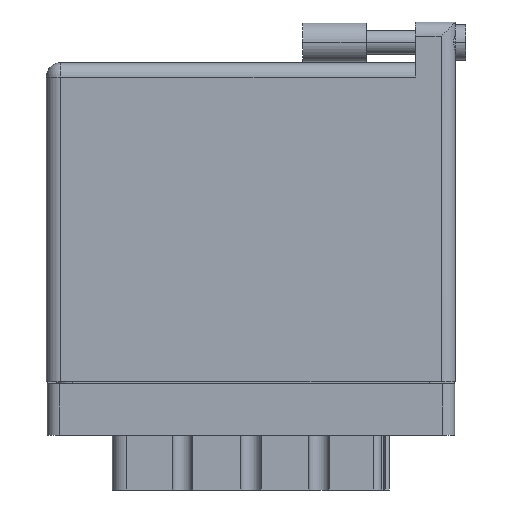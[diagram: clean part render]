
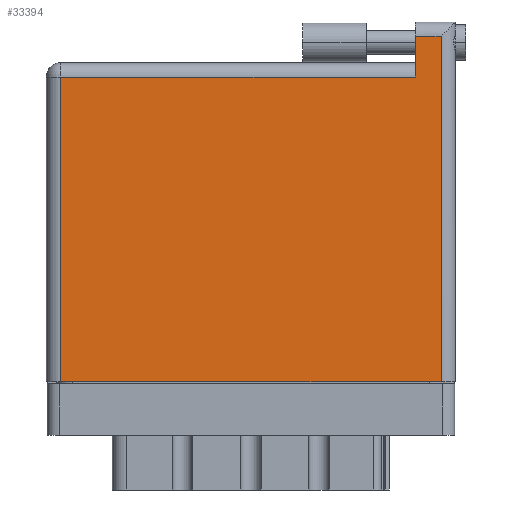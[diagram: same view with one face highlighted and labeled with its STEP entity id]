
A CAD part, front view. The second image highlights one B-rep face of the part: STEP entity #33394.
In plain terms, the highlighted face is planar.
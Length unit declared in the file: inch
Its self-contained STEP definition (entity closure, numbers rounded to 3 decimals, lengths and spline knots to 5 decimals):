
#1506 = DIRECTION ( 'NONE',  ( -1., 0., 0. ) ) ;
#2133 = CARTESIAN_POINT ( 'NONE',  ( 0.07, 0., 0. ) ) ;
#2409 = CARTESIAN_POINT ( 'NONE',  ( 0.07, 1.496, 0. ) ) ;
#3100 = AXIS2_PLACEMENT_3D ( 'NONE', #13180, #16184, #10576 ) ;
#3564 = VERTEX_POINT ( 'NONE', #29487 ) ;
#3925 = VECTOR ( 'NONE', #17186, 39.37008 ) ;
#4521 = ORIENTED_EDGE ( 'NONE', *, *, #5696, .T. ) ;
#5093 = CARTESIAN_POINT ( 'NONE',  ( 1.811, 1.766, 0. ) ) ;
#5696 = EDGE_CURVE ( 'NONE', #34384, #31075, #9668, .T. ) ;
#5845 = VERTEX_POINT ( 'NONE', #22641 ) ;
#6347 = VECTOR ( 'NONE', #23750, 39.37008 ) ;
#7168 = DIRECTION ( 'NONE',  ( -1., 0., 0. ) ) ;
#7696 = VECTOR ( 'NONE', #31211, 39.37008 ) ;
#9415 = VECTOR ( 'NONE', #7168, 39.37008 ) ;
#9668 = LINE ( 'NONE', #19172, #15925 ) ;
#10206 = PLANE ( 'NONE',  #3100 ) ;
#10576 = DIRECTION ( 'NONE',  ( -1., 0., 0. ) ) ;
#13180 = CARTESIAN_POINT ( 'NONE',  ( 0., 1.566, 0. ) ) ;
#14721 = CARTESIAN_POINT ( 'NONE',  ( 1.938, 1.696, 0. ) ) ;
#14875 = LINE ( 'NONE', #24082, #33535 ) ;
#15925 = VECTOR ( 'NONE', #36089, 39.37008 ) ;
#16184 = DIRECTION ( 'NONE',  ( 0., 0., -1. ) ) ;
#17186 = DIRECTION ( 'NONE',  ( 1., 0., 0. ) ) ;
#19172 = CARTESIAN_POINT ( 'NONE',  ( 0.07, 0., 0. ) ) ;
#19460 = ORIENTED_EDGE ( 'NONE', *, *, #34209, .T. ) ;
#20539 = EDGE_CURVE ( 'NONE', #21911, #34384, #14875, .T. ) ;
#21175 = FACE_OUTER_BOUND ( 'NONE', #33820, .T. ) ;
#21911 = VERTEX_POINT ( 'NONE', #26838 ) ;
#22305 = VERTEX_POINT ( 'NONE', #14721 ) ;
#22641 = CARTESIAN_POINT ( 'NONE',  ( 1.938, 0., 0. ) ) ;
#22889 = LINE ( 'NONE', #5093, #7696 ) ;
#23346 = ORIENTED_EDGE ( 'NONE', *, *, #26032, .T. ) ;
#23750 = DIRECTION ( 'NONE',  ( 0., 1., 0. ) ) ;
#24021 = ORIENTED_EDGE ( 'NONE', *, *, #20539, .T. ) ;
#24082 = CARTESIAN_POINT ( 'NONE',  ( 0., 1.496, 0. ) ) ;
#25895 = CARTESIAN_POINT ( 'NONE',  ( 0., 0., 0. ) ) ;
#26032 = EDGE_CURVE ( 'NONE', #31075, #5845, #26668, .T. ) ;
#26668 = LINE ( 'NONE', #25895, #3925 ) ;
#26838 = CARTESIAN_POINT ( 'NONE',  ( 1.811, 1.496, 0. ) ) ;
#26971 = CARTESIAN_POINT ( 'NONE',  ( 1.938, 1.766, 0. ) ) ;
#28850 = ORIENTED_EDGE ( 'NONE', *, *, #34998, .T. ) ;
#29487 = CARTESIAN_POINT ( 'NONE',  ( 1.811, 1.696, 0. ) ) ;
#29806 = CARTESIAN_POINT ( 'NONE',  ( 0., 1.696, 0. ) ) ;
#30067 = LINE ( 'NONE', #26971, #6347 ) ;
#31075 = VERTEX_POINT ( 'NONE', #2133 ) ;
#31211 = DIRECTION ( 'NONE',  ( 0., -1., 0. ) ) ;
#33157 = ORIENTED_EDGE ( 'NONE', *, *, #35463, .T. ) ;
#33394 = ADVANCED_FACE ( 'NONE', ( #21175 ), #10206, .F. ) ;
#33535 = VECTOR ( 'NONE', #1506, 39.37008 ) ;
#33820 = EDGE_LOOP ( 'NONE', ( #23346, #19460, #33157, #28850, #24021, #4521 ) ) ;
#34209 = EDGE_CURVE ( 'NONE', #5845, #22305, #30067, .T. ) ;
#34384 = VERTEX_POINT ( 'NONE', #2409 ) ;
#34998 = EDGE_CURVE ( 'NONE', #3564, #21911, #22889, .T. ) ;
#35463 = EDGE_CURVE ( 'NONE', #22305, #3564, #35727, .T. ) ;
#35727 = LINE ( 'NONE', #29806, #9415 ) ;
#36089 = DIRECTION ( 'NONE',  ( 0., -1., 0. ) ) ;
